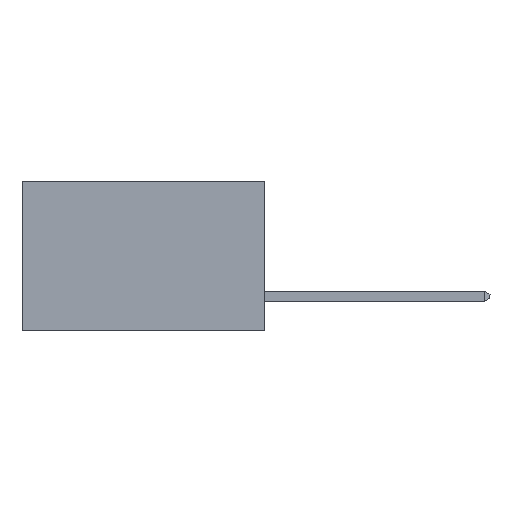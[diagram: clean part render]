
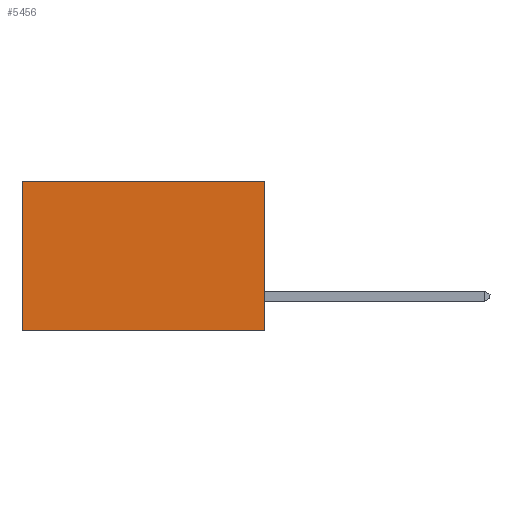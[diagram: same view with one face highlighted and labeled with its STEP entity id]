
A CAD part, left-side view. The second image highlights one B-rep face of the part: STEP entity #5456.
In plain terms, the highlighted planar face has unit normal (-1, 0, 0).
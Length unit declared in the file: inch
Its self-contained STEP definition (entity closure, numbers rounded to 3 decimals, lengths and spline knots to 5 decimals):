
#114 = PLANE ( 'NONE',  #4272 ) ;
#517 = LINE ( 'NONE', #5751, #7702 ) ;
#546 = VERTEX_POINT ( 'NONE', #3399 ) ;
#633 = VECTOR ( 'NONE', #7424, 39.37008 ) ;
#668 = LINE ( 'NONE', #6637, #633 ) ;
#734 = LINE ( 'NONE', #3363, #7909 ) ;
#855 = CARTESIAN_POINT ( 'NONE',  ( 0.2615, 0., -0.37 ) ) ;
#1007 = DIRECTION ( 'NONE',  ( 0., 1., 0. ) ) ;
#2088 = DIRECTION ( 'NONE',  ( 0., 1., 0. ) ) ;
#2452 = EDGE_LOOP ( 'NONE', ( #4523, #5249, #7332, #3400 ) ) ;
#3245 = CARTESIAN_POINT ( 'NONE',  ( 0.2615, 0., 0. ) ) ;
#3272 = VERTEX_POINT ( 'NONE', #4340 ) ;
#3363 = CARTESIAN_POINT ( 'NONE',  ( 0.2615, 0.6, -0.37 ) ) ;
#3399 = CARTESIAN_POINT ( 'NONE',  ( 0.2615, 0., -0.37 ) ) ;
#3400 = ORIENTED_EDGE ( 'NONE', *, *, #6071, .T. ) ;
#3584 = VERTEX_POINT ( 'NONE', #4185 ) ;
#4185 = CARTESIAN_POINT ( 'NONE',  ( 0.2615, 0.6, 0. ) ) ;
#4272 = AXIS2_PLACEMENT_3D ( 'NONE', #855, #6043, #5383 ) ;
#4276 = VECTOR ( 'NONE', #2088, 39.37008 ) ;
#4340 = CARTESIAN_POINT ( 'NONE',  ( 0.2615, 0.6, -0.37 ) ) ;
#4523 = ORIENTED_EDGE ( 'NONE', *, *, #8228, .T. ) ;
#4641 = LINE ( 'NONE', #3245, #4276 ) ;
#4702 = EDGE_CURVE ( 'NONE', #6501, #546, #668, .T. ) ;
#5249 = ORIENTED_EDGE ( 'NONE', *, *, #6277, .F. ) ;
#5383 = DIRECTION ( 'NONE',  ( 0., 0., -1. ) ) ;
#5456 = ADVANCED_FACE ( 'NONE', ( #6607 ), #114, .F. ) ;
#5751 = CARTESIAN_POINT ( 'NONE',  ( 0.2615, 0., -0.37 ) ) ;
#6043 = DIRECTION ( 'NONE',  ( 1., 0., 0. ) ) ;
#6071 = EDGE_CURVE ( 'NONE', #6501, #3584, #4641, .T. ) ;
#6277 = EDGE_CURVE ( 'NONE', #546, #3272, #517, .T. ) ;
#6478 = DIRECTION ( 'NONE',  ( 0., 0., -1. ) ) ;
#6501 = VERTEX_POINT ( 'NONE', #7191 ) ;
#6607 = FACE_OUTER_BOUND ( 'NONE', #2452, .T. ) ;
#6637 = CARTESIAN_POINT ( 'NONE',  ( 0.2615, 0., -0.37 ) ) ;
#7191 = CARTESIAN_POINT ( 'NONE',  ( 0.2615, 0., 0. ) ) ;
#7332 = ORIENTED_EDGE ( 'NONE', *, *, #4702, .F. ) ;
#7424 = DIRECTION ( 'NONE',  ( 0., 0., -1. ) ) ;
#7702 = VECTOR ( 'NONE', #1007, 39.37008 ) ;
#7909 = VECTOR ( 'NONE', #6478, 39.37008 ) ;
#8228 = EDGE_CURVE ( 'NONE', #3584, #3272, #734, .T. ) ;
